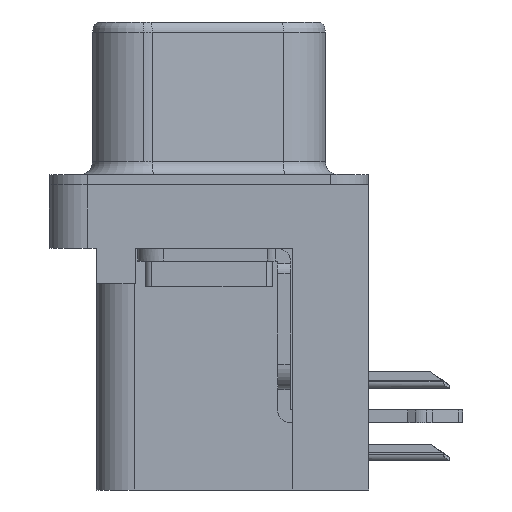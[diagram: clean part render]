
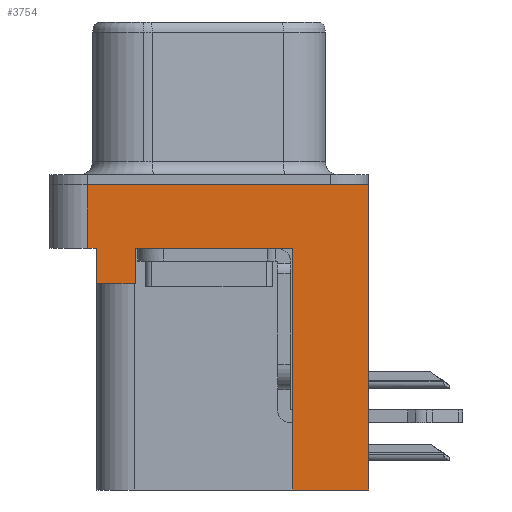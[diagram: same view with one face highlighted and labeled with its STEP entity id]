
A CAD part, left-side view. The second image highlights one B-rep face of the part: STEP entity #3754.
In plain terms, the highlighted planar face has unit normal (-1, 0, 0).
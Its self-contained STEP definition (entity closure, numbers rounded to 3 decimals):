
#97 = EDGE_CURVE ( 'NONE', #1474, #14612, #3596, .T. ) ;
#163 = CARTESIAN_POINT ( 'NONE',  ( -3., -6.275, -2.5 ) ) ;
#309 = ORIENTED_EDGE ( 'NONE', *, *, #20755, .T. ) ;
#688 = LINE ( 'NONE', #8366, #7011 ) ;
#1110 = ORIENTED_EDGE ( 'NONE', *, *, #18830, .F. ) ;
#1474 = VERTEX_POINT ( 'NONE', #8790 ) ;
#1662 = LINE ( 'NONE', #4421, #6474 ) ;
#2401 = VERTEX_POINT ( 'NONE', #6870 ) ;
#2455 = LINE ( 'NONE', #4335, #14584 ) ;
#2911 = DIRECTION ( 'NONE',  ( 0., 1., 0. ) ) ;
#3022 = CARTESIAN_POINT ( 'NONE',  ( -3., 4.425, -2.5 ) ) ;
#3043 = EDGE_CURVE ( 'NONE', #10122, #6537, #2455, .T. ) ;
#3198 = VECTOR ( 'NONE', #8585, 1000. ) ;
#3559 = CARTESIAN_POINT ( 'NONE',  ( -3., -6.275, 0. ) ) ;
#3596 = LINE ( 'NONE', #9374, #12170 ) ;
#3754 = ADVANCED_FACE ( 'NONE', ( #13758 ), #8229, .T. ) ;
#4196 = CARTESIAN_POINT ( 'NONE',  ( -3., -6.275, -12. ) ) ;
#4267 = CARTESIAN_POINT ( 'NONE',  ( -3., -6.275, 0. ) ) ;
#4335 = CARTESIAN_POINT ( 'NONE',  ( -3., -3.295, -12. ) ) ;
#4421 = CARTESIAN_POINT ( 'NONE',  ( -3., 4.775, -2.5 ) ) ;
#4971 = VERTEX_POINT ( 'NONE', #9699 ) ;
#5287 = ORIENTED_EDGE ( 'NONE', *, *, #16080, .T. ) ;
#5646 = VERTEX_POINT ( 'NONE', #4267 ) ;
#6412 = ORIENTED_EDGE ( 'NONE', *, *, #19199, .F. ) ;
#6414 = LINE ( 'NONE', #3559, #14004 ) ;
#6474 = VECTOR ( 'NONE', #13899, 1000. ) ;
#6537 = VERTEX_POINT ( 'NONE', #16530 ) ;
#6870 = CARTESIAN_POINT ( 'NONE',  ( -3., 4.775, 0. ) ) ;
#6981 = DIRECTION ( 'NONE',  ( 0., -1., 0. ) ) ;
#7011 = VECTOR ( 'NONE', #13398, 1000. ) ;
#7308 = EDGE_CURVE ( 'NONE', #10122, #5646, #20933, .T. ) ;
#7492 = DIRECTION ( 'NONE',  ( 0., 1., 0. ) ) ;
#7710 = CARTESIAN_POINT ( 'NONE',  ( -3., 4.775, -2.5 ) ) ;
#8229 = PLANE ( 'NONE',  #20206 ) ;
#8366 = CARTESIAN_POINT ( 'NONE',  ( -3., 2.895, -3.9 ) ) ;
#8408 = ORIENTED_EDGE ( 'NONE', *, *, #14484, .T. ) ;
#8585 = DIRECTION ( 'NONE',  ( 0., 0., 1. ) ) ;
#8790 = CARTESIAN_POINT ( 'NONE',  ( -3., 4.425, -3.9 ) ) ;
#9374 = CARTESIAN_POINT ( 'NONE',  ( -3., 4.425, -3.9 ) ) ;
#9528 = CARTESIAN_POINT ( 'NONE',  ( -3., -6.275, -2.5 ) ) ;
#9674 = VECTOR ( 'NONE', #6981, 1000. ) ;
#9699 = CARTESIAN_POINT ( 'NONE',  ( -3., -3.295, -2.5 ) ) ;
#9807 = CARTESIAN_POINT ( 'NONE',  ( -3., -3.295, -12. ) ) ;
#10122 = VERTEX_POINT ( 'NONE', #4196 ) ;
#10124 = LINE ( 'NONE', #9807, #15730 ) ;
#10291 = EDGE_CURVE ( 'NONE', #6537, #4971, #10124, .T. ) ;
#10526 = LINE ( 'NONE', #13425, #16880 ) ;
#11303 = ORIENTED_EDGE ( 'NONE', *, *, #97, .F. ) ;
#11795 = ORIENTED_EDGE ( 'NONE', *, *, #7308, .T. ) ;
#11836 = EDGE_CURVE ( 'NONE', #20159, #2401, #1662, .T. ) ;
#12170 = VECTOR ( 'NONE', #20711, 1000. ) ;
#13056 = DIRECTION ( 'NONE',  ( 0., 0., 1. ) ) ;
#13398 = DIRECTION ( 'NONE',  ( 0., 0., 1. ) ) ;
#13425 = CARTESIAN_POINT ( 'NONE',  ( -3., -6.275, -2.5 ) ) ;
#13758 = FACE_OUTER_BOUND ( 'NONE', #20402, .T. ) ;
#13899 = DIRECTION ( 'NONE',  ( 0., 0., 1. ) ) ;
#13978 = LINE ( 'NONE', #16631, #9674 ) ;
#14004 = VECTOR ( 'NONE', #19440, 1000. ) ;
#14072 = CARTESIAN_POINT ( 'NONE',  ( -3., 4.425, -3.9 ) ) ;
#14484 = EDGE_CURVE ( 'NONE', #18548, #4971, #10526, .T. ) ;
#14539 = DIRECTION ( 'NONE',  ( 0., 0., 1. ) ) ;
#14584 = VECTOR ( 'NONE', #7492, 1000. ) ;
#14612 = VERTEX_POINT ( 'NONE', #3022 ) ;
#15015 = VECTOR ( 'NONE', #2911, 1000. ) ;
#15676 = CARTESIAN_POINT ( 'NONE',  ( -3., 2.895, -2.5 ) ) ;
#15730 = VECTOR ( 'NONE', #13056, 1000. ) ;
#15985 = VERTEX_POINT ( 'NONE', #17683 ) ;
#16080 = EDGE_CURVE ( 'NONE', #20159, #14612, #13978, .T. ) ;
#16251 = DIRECTION ( 'NONE',  ( -1., 0., 0. ) ) ;
#16294 = ORIENTED_EDGE ( 'NONE', *, *, #10291, .F. ) ;
#16530 = CARTESIAN_POINT ( 'NONE',  ( -3., -3.295, -12. ) ) ;
#16631 = CARTESIAN_POINT ( 'NONE',  ( -3., -6.275, -2.5 ) ) ;
#16755 = DIRECTION ( 'NONE',  ( 0., -1., 0. ) ) ;
#16880 = VECTOR ( 'NONE', #16755, 1000. ) ;
#17336 = ORIENTED_EDGE ( 'NONE', *, *, #11836, .F. ) ;
#17578 = ORIENTED_EDGE ( 'NONE', *, *, #3043, .F. ) ;
#17683 = CARTESIAN_POINT ( 'NONE',  ( -3., 2.895, -3.9 ) ) ;
#18548 = VERTEX_POINT ( 'NONE', #15676 ) ;
#18830 = EDGE_CURVE ( 'NONE', #2401, #5646, #6414, .T. ) ;
#19199 = EDGE_CURVE ( 'NONE', #15985, #1474, #19290, .T. ) ;
#19290 = LINE ( 'NONE', #14072, #15015 ) ;
#19440 = DIRECTION ( 'NONE',  ( 0., -1., 0. ) ) ;
#20159 = VERTEX_POINT ( 'NONE', #7710 ) ;
#20206 = AXIS2_PLACEMENT_3D ( 'NONE', #163, #16251, #14539 ) ;
#20402 = EDGE_LOOP ( 'NONE', ( #1110, #17336, #5287, #11303, #6412, #309, #8408, #16294, #17578, #11795 ) ) ;
#20711 = DIRECTION ( 'NONE',  ( 0., 0., 1. ) ) ;
#20755 = EDGE_CURVE ( 'NONE', #15985, #18548, #688, .T. ) ;
#20933 = LINE ( 'NONE', #9528, #3198 ) ;
